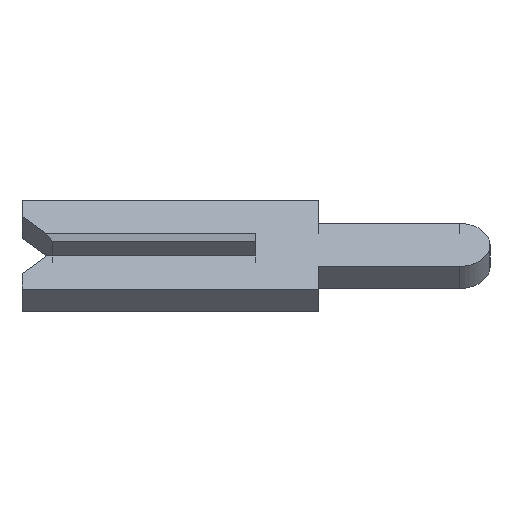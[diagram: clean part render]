
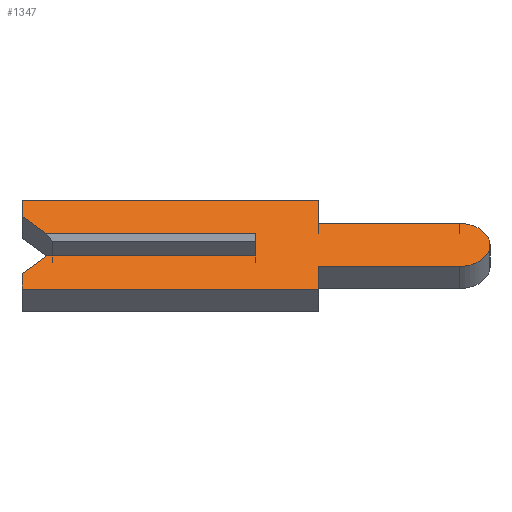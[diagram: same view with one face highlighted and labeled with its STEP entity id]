
A CAD part, left-side view. The second image highlights one B-rep face of the part: STEP entity #1347.
In plain terms, the highlighted face is planar.
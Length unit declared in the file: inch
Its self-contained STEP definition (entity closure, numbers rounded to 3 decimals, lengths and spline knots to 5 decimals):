
#31 = CARTESIAN_POINT ( 'NONE',  ( -0.01, 0.134, -0.01 ) ) ;
#33 = CARTESIAN_POINT ( 'NONE',  ( -0.01, -0.04, -0.04 ) ) ;
#36 = CARTESIAN_POINT ( 'NONE',  ( -0.01, -0.1305, -0.0195 ) ) ;
#42 = ORIENTED_EDGE ( 'NONE', *, *, #235, .F. ) ;
#47 = VECTOR ( 'NONE', #159, 39.37008 ) ;
#55 = ORIENTED_EDGE ( 'NONE', *, *, #132, .F. ) ;
#62 = DIRECTION ( 'NONE',  ( 1., 0., 0. ) ) ;
#66 = VECTOR ( 'NONE', #569, 39.37008 ) ;
#79 = EDGE_CURVE ( 'NONE', #84, #692, #785, .T. ) ;
#84 = VERTEX_POINT ( 'NONE', #1130 ) ;
#92 = CARTESIAN_POINT ( 'NONE',  ( -0.01, -0.1305, -0.01 ) ) ;
#116 = CARTESIAN_POINT ( 'NONE',  ( -0.01, 0.15, 0.026 ) ) ;
#118 = DIRECTION ( 'NONE',  ( 0., -1., 0. ) ) ;
#132 = EDGE_CURVE ( 'NONE', #886, #995, #317, .T. ) ;
#159 = DIRECTION ( 'NONE',  ( 0., 0., 1. ) ) ;
#174 = CARTESIAN_POINT ( 'NONE',  ( -0.01, -0.04, 0.0195 ) ) ;
#185 = LINE ( 'NONE', #1083, #66 ) ;
#194 = CARTESIAN_POINT ( 'NONE',  ( -0.01, -0.04, 0.04 ) ) ;
#205 = VECTOR ( 'NONE', #254, 39.37008 ) ;
#216 = LINE ( 'NONE', #194, #818 ) ;
#222 = VERTEX_POINT ( 'NONE', #1135 ) ;
#235 = EDGE_CURVE ( 'NONE', #849, #1309, #216, .T. ) ;
#239 = ORIENTED_EDGE ( 'NONE', *, *, #79, .F. ) ;
#243 = LINE ( 'NONE', #343, #205 ) ;
#254 = DIRECTION ( 'NONE',  ( 0., 0., 1. ) ) ;
#255 = LINE ( 'NONE', #544, #1346 ) ;
#269 = VECTOR ( 'NONE', #676, 39.37008 ) ;
#270 = EDGE_CURVE ( 'NONE', #1342, #886, #1019, .T. ) ;
#280 = ORIENTED_EDGE ( 'NONE', *, *, #1280, .F. ) ;
#285 = ORIENTED_EDGE ( 'NONE', *, *, #523, .F. ) ;
#295 = VERTEX_POINT ( 'NONE', #299 ) ;
#299 = CARTESIAN_POINT ( 'NONE',  ( -0.01, 0.15, -0.04 ) ) ;
#313 = DIRECTION ( 'NONE',  ( 0., -1., 0. ) ) ;
#317 = LINE ( 'NONE', #92, #576 ) ;
#334 = CARTESIAN_POINT ( 'NONE',  ( -0.01, 0.15, -0.04 ) ) ;
#343 = CARTESIAN_POINT ( 'NONE',  ( -0.01, 0., 0.0065 ) ) ;
#344 = FACE_OUTER_BOUND ( 'NONE', #366, .T. ) ;
#366 = EDGE_LOOP ( 'NONE', ( #1242, #813, #55, #561, #393, #1119, #787, #280, #239, #1143, #42, #285, #1220, #537 ) ) ;
#382 = VECTOR ( 'NONE', #821, 39.37008 ) ;
#385 = DIRECTION ( 'NONE',  ( 0., 0., -1. ) ) ;
#393 = ORIENTED_EDGE ( 'NONE', *, *, #1121, .F. ) ;
#422 = CARTESIAN_POINT ( 'NONE',  ( -0.01, 0.1305, -0.0065 ) ) ;
#428 = VERTEX_POINT ( 'NONE', #116 ) ;
#466 = VERTEX_POINT ( 'NONE', #1298 ) ;
#472 = CARTESIAN_POINT ( 'NONE',  ( -0.01, 0.15, -0.026 ) ) ;
#487 = AXIS2_PLACEMENT_3D ( 'NONE', #1343, #704, #1370 ) ;
#523 = EDGE_CURVE ( 'NONE', #811, #849, #618, .T. ) ;
#537 = ORIENTED_EDGE ( 'NONE', *, *, #1075, .F. ) ;
#544 = CARTESIAN_POINT ( 'NONE',  ( -0.01, 0.15, 0.026 ) ) ;
#561 = ORIENTED_EDGE ( 'NONE', *, *, #270, .F. ) ;
#564 = LINE ( 'NONE', #334, #269 ) ;
#569 = DIRECTION ( 'NONE',  ( 0., 0., -1. ) ) ;
#576 = VECTOR ( 'NONE', #313, 39.37008 ) ;
#593 = CARTESIAN_POINT ( 'NONE',  ( -0.01, 0.15, 0.01 ) ) ;
#618 = LINE ( 'NONE', #1065, #1059 ) ;
#623 = EDGE_CURVE ( 'NONE', #428, #811, #255, .T. ) ;
#626 = LINE ( 'NONE', #472, #47 ) ;
#666 = CARTESIAN_POINT ( 'NONE',  ( -0.01, 0., -0.01 ) ) ;
#670 = CARTESIAN_POINT ( 'NONE',  ( -0.01, -0.04, 0.04 ) ) ;
#676 = DIRECTION ( 'NONE',  ( 0., 1., 0. ) ) ;
#692 = VERTEX_POINT ( 'NONE', #36 ) ;
#699 = DIRECTION ( 'NONE',  ( 0., -1., 0. ) ) ;
#704 = DIRECTION ( 'NONE',  ( 1., 0., 0. ) ) ;
#705 = VECTOR ( 'NONE', #1223, 39.37008 ) ;
#712 = LINE ( 'NONE', #1324, #1036 ) ;
#721 = AXIS2_PLACEMENT_3D ( 'NONE', #1037, #62, #385 ) ;
#722 = DIRECTION ( 'NONE',  ( 0., 0., -1. ) ) ;
#731 = EDGE_CURVE ( 'NONE', #884, #295, #564, .T. ) ;
#761 = VECTOR ( 'NONE', #790, 39.37008 ) ;
#780 = CARTESIAN_POINT ( 'NONE',  ( -0.01, 0.15, 0.04 ) ) ;
#785 = CIRCLE ( 'NONE', #487, 0.0195 ) ;
#787 = ORIENTED_EDGE ( 'NONE', *, *, #940, .F. ) ;
#790 = DIRECTION ( 'NONE',  ( 0., -1., 0. ) ) ;
#811 = VERTEX_POINT ( 'NONE', #780 ) ;
#813 = ORIENTED_EDGE ( 'NONE', *, *, #899, .F. ) ;
#818 = VECTOR ( 'NONE', #722, 39.37008 ) ;
#821 = DIRECTION ( 'NONE',  ( 0., 0.707, 0.707 ) ) ;
#849 = VERTEX_POINT ( 'NONE', #670 ) ;
#867 = DIRECTION ( 'NONE',  ( 0., 0., 1. ) ) ;
#884 = VERTEX_POINT ( 'NONE', #33 ) ;
#886 = VERTEX_POINT ( 'NONE', #31 ) ;
#899 = EDGE_CURVE ( 'NONE', #995, #466, #243, .T. ) ;
#914 = CARTESIAN_POINT ( 'NONE',  ( -0.01, -0.04, -0.0195 ) ) ;
#940 = EDGE_CURVE ( 'NONE', #1215, #884, #185, .T. ) ;
#995 = VERTEX_POINT ( 'NONE', #666 ) ;
#1011 = EDGE_CURVE ( 'NONE', #1309, #84, #712, .T. ) ;
#1019 = LINE ( 'NONE', #422, #1368 ) ;
#1021 = CARTESIAN_POINT ( 'NONE',  ( -0.01, 0.15, -0.026 ) ) ;
#1036 = VECTOR ( 'NONE', #699, 39.37008 ) ;
#1037 = CARTESIAN_POINT ( 'NONE',  ( -0.01, -0.1305, 0. ) ) ;
#1059 = VECTOR ( 'NONE', #118, 39.37008 ) ;
#1065 = CARTESIAN_POINT ( 'NONE',  ( -0.01, 0.15, 0.04 ) ) ;
#1075 = EDGE_CURVE ( 'NONE', #222, #428, #1289, .T. ) ;
#1083 = CARTESIAN_POINT ( 'NONE',  ( -0.01, -0.04, -0.04 ) ) ;
#1110 = CARTESIAN_POINT ( 'NONE',  ( -0.01, -0.04, -0.0195 ) ) ;
#1119 = ORIENTED_EDGE ( 'NONE', *, *, #731, .F. ) ;
#1121 = EDGE_CURVE ( 'NONE', #295, #1342, #626, .T. ) ;
#1130 = CARTESIAN_POINT ( 'NONE',  ( -0.01, -0.1305, 0.0195 ) ) ;
#1135 = CARTESIAN_POINT ( 'NONE',  ( -0.01, 0.134, 0.01 ) ) ;
#1139 = CARTESIAN_POINT ( 'NONE',  ( -0.01, 0.1305, 0.0065 ) ) ;
#1143 = ORIENTED_EDGE ( 'NONE', *, *, #1011, .F. ) ;
#1146 = DIRECTION ( 'NONE',  ( 0., -0.707, 0.707 ) ) ;
#1159 = EDGE_CURVE ( 'NONE', #222, #466, #1238, .T. ) ;
#1215 = VERTEX_POINT ( 'NONE', #914 ) ;
#1220 = ORIENTED_EDGE ( 'NONE', *, *, #623, .F. ) ;
#1223 = DIRECTION ( 'NONE',  ( 0., 1., 0. ) ) ;
#1238 = LINE ( 'NONE', #593, #761 ) ;
#1242 = ORIENTED_EDGE ( 'NONE', *, *, #1159, .T. ) ;
#1250 = LINE ( 'NONE', #1110, #705 ) ;
#1280 = EDGE_CURVE ( 'NONE', #692, #1215, #1250, .T. ) ;
#1289 = LINE ( 'NONE', #1139, #382 ) ;
#1298 = CARTESIAN_POINT ( 'NONE',  ( -0.01, 0., 0.01 ) ) ;
#1309 = VERTEX_POINT ( 'NONE', #174 ) ;
#1324 = CARTESIAN_POINT ( 'NONE',  ( -0.01, -0.04, 0.0195 ) ) ;
#1342 = VERTEX_POINT ( 'NONE', #1021 ) ;
#1343 = CARTESIAN_POINT ( 'NONE',  ( -0.01, -0.1305, 0. ) ) ;
#1346 = VECTOR ( 'NONE', #867, 39.37008 ) ;
#1347 = ADVANCED_FACE ( 'NONE', ( #344 ), #1350, .F. ) ;
#1350 = PLANE ( 'NONE',  #721 ) ;
#1368 = VECTOR ( 'NONE', #1146, 39.37008 ) ;
#1370 = DIRECTION ( 'NONE',  ( 0., 0., -1. ) ) ;
